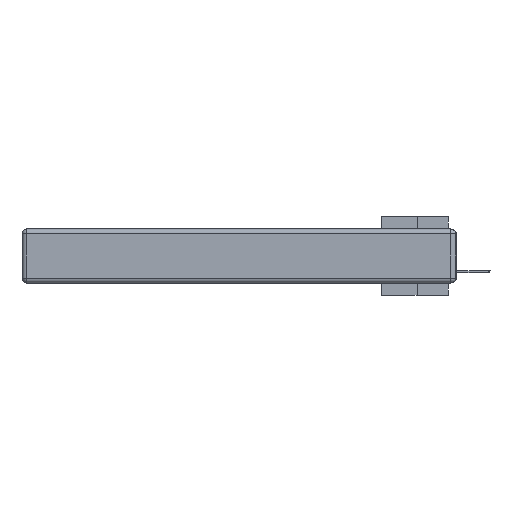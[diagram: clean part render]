
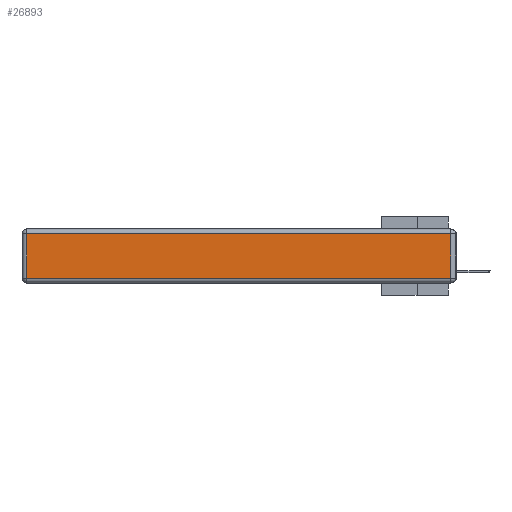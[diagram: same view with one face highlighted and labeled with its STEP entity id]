
A CAD part, left-side view. The second image highlights one B-rep face of the part: STEP entity #26893.
In plain terms, the highlighted planar face has unit normal (-1, 0, 0).
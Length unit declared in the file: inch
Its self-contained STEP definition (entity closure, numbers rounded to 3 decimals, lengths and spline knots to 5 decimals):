
#295 = EDGE_CURVE ( 'NONE', #12389, #6791, #8021, .T. ) ;
#1223 = DIRECTION ( 'NONE',  ( 0., 0., -1. ) ) ;
#1929 = EDGE_CURVE ( 'NONE', #26163, #12389, #30112, .T. ) ;
#2726 = ORIENTED_EDGE ( 'NONE', *, *, #9717, .T. ) ;
#4695 = VERTEX_POINT ( 'NONE', #11643 ) ;
#4915 = LINE ( 'NONE', #14061, #19215 ) ;
#6301 = VECTOR ( 'NONE', #20422, 39.37008 ) ;
#6791 = VERTEX_POINT ( 'NONE', #28620 ) ;
#8021 = LINE ( 'NONE', #17564, #6301 ) ;
#9717 = EDGE_CURVE ( 'NONE', #6791, #4695, #4915, .T. ) ;
#11643 = CARTESIAN_POINT ( 'NONE',  ( 0., 2.72, -0.03 ) ) ;
#12274 = EDGE_CURVE ( 'NONE', #4695, #26163, #17081, .T. ) ;
#12389 = VERTEX_POINT ( 'NONE', #39850 ) ;
#13604 = CARTESIAN_POINT ( 'NONE',  ( 0., 2.72, -0.313 ) ) ;
#13664 = ORIENTED_EDGE ( 'NONE', *, *, #295, .T. ) ;
#14061 = CARTESIAN_POINT ( 'NONE',  ( 0., 2.75, -0.03 ) ) ;
#14484 = CARTESIAN_POINT ( 'NONE',  ( 0., 0., -0.313 ) ) ;
#14600 = AXIS2_PLACEMENT_3D ( 'NONE', #29694, #17298, #39062 ) ;
#14667 = PLANE ( 'NONE',  #14600 ) ;
#17081 = LINE ( 'NONE', #39046, #39398 ) ;
#17298 = DIRECTION ( 'NONE',  ( -1., 0., 0. ) ) ;
#17564 = CARTESIAN_POINT ( 'NONE',  ( 0., 0.03, -0.343 ) ) ;
#19215 = VECTOR ( 'NONE', #29695, 39.37008 ) ;
#20422 = DIRECTION ( 'NONE',  ( 0., 0., 1. ) ) ;
#21481 = ORIENTED_EDGE ( 'NONE', *, *, #1929, .T. ) ;
#26163 = VERTEX_POINT ( 'NONE', #13604 ) ;
#26248 = FACE_OUTER_BOUND ( 'NONE', #28655, .T. ) ;
#26893 = ADVANCED_FACE ( 'NONE', ( #26248 ), #14667, .T. ) ;
#28620 = CARTESIAN_POINT ( 'NONE',  ( 0., 0.03, -0.03 ) ) ;
#28655 = EDGE_LOOP ( 'NONE', ( #21481, #13664, #2726, #36644 ) ) ;
#29694 = CARTESIAN_POINT ( 'NONE',  ( 0., 0., -0.343 ) ) ;
#29695 = DIRECTION ( 'NONE',  ( 0., 1., 0. ) ) ;
#30112 = LINE ( 'NONE', #14484, #31911 ) ;
#31911 = VECTOR ( 'NONE', #32969, 39.37008 ) ;
#32969 = DIRECTION ( 'NONE',  ( 0., -1., 0. ) ) ;
#36644 = ORIENTED_EDGE ( 'NONE', *, *, #12274, .T. ) ;
#39046 = CARTESIAN_POINT ( 'NONE',  ( 0., 2.72, -0.343 ) ) ;
#39062 = DIRECTION ( 'NONE',  ( 0., 0., 1. ) ) ;
#39398 = VECTOR ( 'NONE', #1223, 39.37008 ) ;
#39850 = CARTESIAN_POINT ( 'NONE',  ( 0., 0.03, -0.313 ) ) ;
